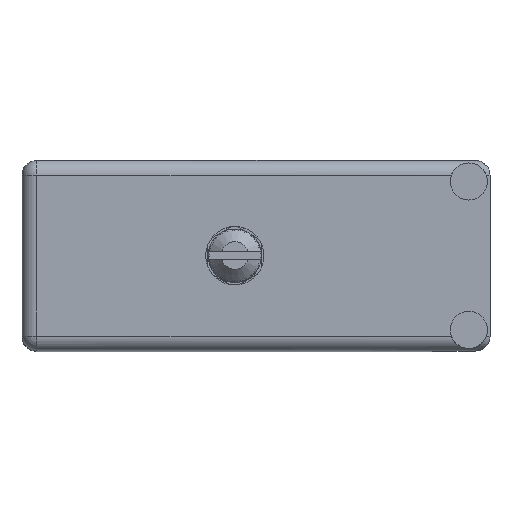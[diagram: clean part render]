
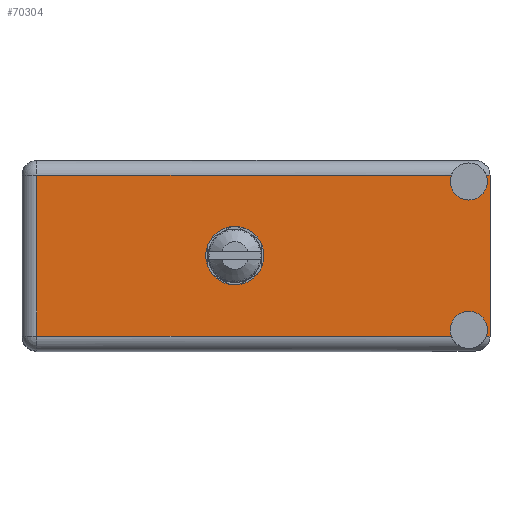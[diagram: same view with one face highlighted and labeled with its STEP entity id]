
A CAD part, top view. The second image highlights one B-rep face of the part: STEP entity #70304.
In plain terms, the highlighted face is planar.
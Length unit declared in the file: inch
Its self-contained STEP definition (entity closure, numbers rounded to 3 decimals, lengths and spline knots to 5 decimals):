
#731 = AXIS2_PLACEMENT_3D ( 'NONE', #25473, #57731, #17039 ) ;
#4222 = PLANE ( 'NONE',  #97793 ) ;
#5796 = EDGE_CURVE ( 'NONE', #47540, #18841, #63016, .T. ) ;
#7928 = EDGE_LOOP ( 'NONE', ( #30374, #60024 ) ) ;
#7939 = ORIENTED_EDGE ( 'NONE', *, *, #38217, .T. ) ;
#9441 = CARTESIAN_POINT ( 'NONE',  ( 2.02562, 1.566, -0.829 ) ) ;
#9527 = AXIS2_PLACEMENT_3D ( 'NONE', #52000, #77223, #100889 ) ;
#10276 = AXIS2_PLACEMENT_3D ( 'NONE', #60321, #50352, #67722 ) ;
#12459 = CIRCLE ( 'NONE', #58002, 0.1375 ) ;
#13651 = FACE_BOUND ( 'NONE', #7928, .T. ) ;
#14657 = CARTESIAN_POINT ( 'NONE',  ( 2.108, 1.566, -0.0995 ) ) ;
#14869 = LINE ( 'NONE', #61883, #51647 ) ;
#15028 = ORIENTED_EDGE ( 'NONE', *, *, #32478, .T. ) ;
#15838 = CIRCLE ( 'NONE', #731, 0.0875 ) ;
#17039 = DIRECTION ( 'NONE',  ( 0., 0., 1. ) ) ;
#18450 = VERTEX_POINT ( 'NONE', #67613 ) ;
#18470 = ORIENTED_EDGE ( 'NONE', *, *, #43752, .T. ) ;
#18841 = VERTEX_POINT ( 'NONE', #25783 ) ;
#21006 = VECTOR ( 'NONE', #50266, 39.37008 ) ;
#21027 = FACE_OUTER_BOUND ( 'NONE', #33410, .T. ) ;
#22429 = AXIS2_PLACEMENT_3D ( 'NONE', #14657, #79543, #87410 ) ;
#23291 = DIRECTION ( 'NONE',  ( 0., 0., 1. ) ) ;
#23626 = VERTEX_POINT ( 'NONE', #38135 ) ;
#24154 = VERTEX_POINT ( 'NONE', #100079 ) ;
#25473 = CARTESIAN_POINT ( 'NONE',  ( 2.108, 1.566, -0.7995 ) ) ;
#25783 = CARTESIAN_POINT ( 'NONE',  ( 1.004, 1.566, -0.587 ) ) ;
#26025 = DIRECTION ( 'NONE',  ( 1., 0., 0. ) ) ;
#26701 = EDGE_CURVE ( 'NONE', #18841, #47540, #12459, .T. ) ;
#26806 = EDGE_CURVE ( 'NONE', #34942, #92852, #15838, .T. ) ;
#30259 = VERTEX_POINT ( 'NONE', #51203 ) ;
#30374 = ORIENTED_EDGE ( 'NONE', *, *, #5796, .F. ) ;
#30890 = VECTOR ( 'NONE', #97271, 39.37008 ) ;
#32478 = EDGE_CURVE ( 'NONE', #103456, #45621, #58702, .T. ) ;
#32495 = VECTOR ( 'NONE', #66993, 39.37008 ) ;
#33410 = EDGE_LOOP ( 'NONE', ( #103243, #70136, #96630, #7939, #80948, #15028, #43004, #73250, #68359, #18470 ) ) ;
#34428 = CARTESIAN_POINT ( 'NONE',  ( 0., 1.566, -0.829 ) ) ;
#34942 = VERTEX_POINT ( 'NONE', #9441 ) ;
#36731 = VERTEX_POINT ( 'NONE', #98530 ) ;
#38135 = CARTESIAN_POINT ( 'NONE',  ( 2.108, 1.566, -0.187 ) ) ;
#38153 = DIRECTION ( 'NONE',  ( -1., 0., 0. ) ) ;
#38217 = EDGE_CURVE ( 'NONE', #36731, #30259, #97222, .T. ) ;
#39702 = DIRECTION ( 'NONE',  ( 0., 1., 0. ) ) ;
#40900 = CARTESIAN_POINT ( 'NONE',  ( 0.07, 1.566, -0.899 ) ) ;
#42207 = CARTESIAN_POINT ( 'NONE',  ( 2.208, 1.566, -0.07 ) ) ;
#43004 = ORIENTED_EDGE ( 'NONE', *, *, #76045, .F. ) ;
#43752 = EDGE_CURVE ( 'NONE', #24154, #18450, #64639, .T. ) ;
#45359 = DIRECTION ( 'NONE',  ( 0., 0., 1. ) ) ;
#45621 = VERTEX_POINT ( 'NONE', #56722 ) ;
#47540 = VERTEX_POINT ( 'NONE', #54801 ) ;
#48295 = CARTESIAN_POINT ( 'NONE',  ( 2.108, 1.566, -0.712 ) ) ;
#49309 = CARTESIAN_POINT ( 'NONE',  ( 2.208, 1.566, -0.07 ) ) ;
#50266 = DIRECTION ( 'NONE',  ( -1., 0., 0. ) ) ;
#50352 = DIRECTION ( 'NONE',  ( 0., 1., 0. ) ) ;
#51203 = CARTESIAN_POINT ( 'NONE',  ( 2.208, 1.566, -0.07 ) ) ;
#51647 = VECTOR ( 'NONE', #38153, 39.37008 ) ;
#51732 = LINE ( 'NONE', #42207, #32495 ) ;
#52000 = CARTESIAN_POINT ( 'NONE',  ( 2.108, 1.566, -0.7995 ) ) ;
#52914 = AXIS2_PLACEMENT_3D ( 'NONE', #56595, #39702, #23291 ) ;
#54518 = CIRCLE ( 'NONE', #22429, 0.0875 ) ;
#54801 = CARTESIAN_POINT ( 'NONE',  ( 1.004, 1.566, -0.312 ) ) ;
#56595 = CARTESIAN_POINT ( 'NONE',  ( 1.004, 1.566, -0.4495 ) ) ;
#56722 = CARTESIAN_POINT ( 'NONE',  ( 2.19038, 1.566, -0.829 ) ) ;
#57731 = DIRECTION ( 'NONE',  ( 0., 1., 0. ) ) ;
#58002 = AXIS2_PLACEMENT_3D ( 'NONE', #74829, #92157, #84264 ) ;
#58702 = LINE ( 'NONE', #34428, #21006 ) ;
#60024 = ORIENTED_EDGE ( 'NONE', *, *, #26701, .F. ) ;
#60321 = CARTESIAN_POINT ( 'NONE',  ( 2.108, 1.566, -0.0995 ) ) ;
#61883 = CARTESIAN_POINT ( 'NONE',  ( 0., 1.566, -0.829 ) ) ;
#63016 = CIRCLE ( 'NONE', #52914, 0.1375 ) ;
#64639 = LINE ( 'NONE', #40900, #30890 ) ;
#65734 = CARTESIAN_POINT ( 'NONE',  ( 2.02562, 1.566, -0.07 ) ) ;
#66192 = VERTEX_POINT ( 'NONE', #65734 ) ;
#66540 = EDGE_CURVE ( 'NONE', #23626, #66192, #102824, .T. ) ;
#66993 = DIRECTION ( 'NONE',  ( 1., 0., 0. ) ) ;
#67613 = CARTESIAN_POINT ( 'NONE',  ( 0.07, 1.566, -0.07 ) ) ;
#67722 = DIRECTION ( 'NONE',  ( 0., 0., 1. ) ) ;
#68359 = ORIENTED_EDGE ( 'NONE', *, *, #100184, .T. ) ;
#70136 = ORIENTED_EDGE ( 'NONE', *, *, #66540, .F. ) ;
#70304 = ADVANCED_FACE ( 'NONE', ( #13651, #21027 ), #4222, .T. ) ;
#73250 = ORIENTED_EDGE ( 'NONE', *, *, #26806, .F. ) ;
#74829 = CARTESIAN_POINT ( 'NONE',  ( 1.004, 1.566, -0.4495 ) ) ;
#75948 = DIRECTION ( 'NONE',  ( 0., 0., 1. ) ) ;
#76045 = EDGE_CURVE ( 'NONE', #92852, #45621, #103736, .T. ) ;
#76109 = VECTOR ( 'NONE', #45359, 39.37008 ) ;
#76429 = LINE ( 'NONE', #78494, #76109 ) ;
#77223 = DIRECTION ( 'NONE',  ( 0., 1., 0. ) ) ;
#78494 = CARTESIAN_POINT ( 'NONE',  ( 2.208, 1.566, 0. ) ) ;
#79543 = DIRECTION ( 'NONE',  ( 0., 1., 0. ) ) ;
#80948 = ORIENTED_EDGE ( 'NONE', *, *, #101682, .F. ) ;
#84264 = DIRECTION ( 'NONE',  ( 0., 0., 1. ) ) ;
#84868 = DIRECTION ( 'NONE',  ( 0., 1., 0. ) ) ;
#85731 = CARTESIAN_POINT ( 'NONE',  ( 2.208, 1.566, -0.829 ) ) ;
#87410 = DIRECTION ( 'NONE',  ( 0., 0., 1. ) ) ;
#91353 = VECTOR ( 'NONE', #26025, 39.37008 ) ;
#92157 = DIRECTION ( 'NONE',  ( 0., 1., 0. ) ) ;
#92852 = VERTEX_POINT ( 'NONE', #48295 ) ;
#94315 = CARTESIAN_POINT ( 'NONE',  ( 0., 1.566, -0.899 ) ) ;
#94467 = EDGE_CURVE ( 'NONE', #18450, #66192, #51732, .T. ) ;
#96630 = ORIENTED_EDGE ( 'NONE', *, *, #97651, .F. ) ;
#97222 = LINE ( 'NONE', #49309, #91353 ) ;
#97271 = DIRECTION ( 'NONE',  ( 0., 0., 1. ) ) ;
#97651 = EDGE_CURVE ( 'NONE', #36731, #23626, #54518, .T. ) ;
#97793 = AXIS2_PLACEMENT_3D ( 'NONE', #94315, #84868, #75948 ) ;
#98530 = CARTESIAN_POINT ( 'NONE',  ( 2.19038, 1.566, -0.07 ) ) ;
#100079 = CARTESIAN_POINT ( 'NONE',  ( 0.07, 1.566, -0.829 ) ) ;
#100184 = EDGE_CURVE ( 'NONE', #34942, #24154, #14869, .T. ) ;
#100889 = DIRECTION ( 'NONE',  ( 0., 0., 1. ) ) ;
#101682 = EDGE_CURVE ( 'NONE', #103456, #30259, #76429, .T. ) ;
#102824 = CIRCLE ( 'NONE', #10276, 0.0875 ) ;
#103243 = ORIENTED_EDGE ( 'NONE', *, *, #94467, .T. ) ;
#103456 = VERTEX_POINT ( 'NONE', #85731 ) ;
#103736 = CIRCLE ( 'NONE', #9527, 0.0875 ) ;
